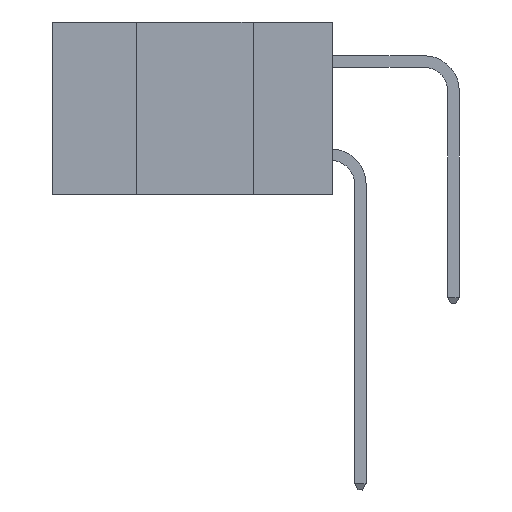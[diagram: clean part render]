
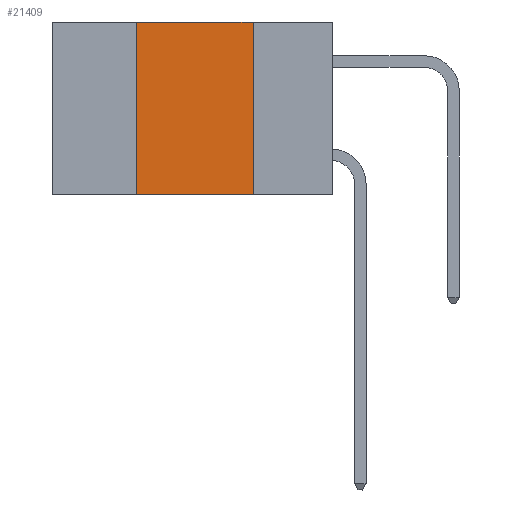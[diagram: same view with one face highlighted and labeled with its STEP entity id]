
A CAD part, left-side view. The second image highlights one B-rep face of the part: STEP entity #21409.
In plain terms, the highlighted planar face has unit normal (-1, 0, 0).
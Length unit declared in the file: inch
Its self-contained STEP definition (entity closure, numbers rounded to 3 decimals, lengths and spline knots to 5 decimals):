
#1539 = DIRECTION ( 'NONE',  ( 0., 0., -1. ) ) ;
#1586 = VERTEX_POINT ( 'NONE', #4110 ) ;
#3507 = ORIENTED_EDGE ( 'NONE', *, *, #20009, .F. ) ;
#4110 = CARTESIAN_POINT ( 'NONE',  ( 0., 0.42, -0.37 ) ) ;
#5303 = CARTESIAN_POINT ( 'NONE',  ( 0., 0.42, 0. ) ) ;
#6192 = ORIENTED_EDGE ( 'NONE', *, *, #22214, .F. ) ;
#6319 = VERTEX_POINT ( 'NONE', #9510 ) ;
#7118 = VECTOR ( 'NONE', #18454, 39.37008 ) ;
#7575 = CARTESIAN_POINT ( 'NONE',  ( 0., 0.6, 0. ) ) ;
#8699 = DIRECTION ( 'NONE',  ( 0., 0., 1. ) ) ;
#8933 = LINE ( 'NONE', #19924, #21434 ) ;
#9510 = CARTESIAN_POINT ( 'NONE',  ( 0., 0.17, -0.37 ) ) ;
#11011 = VERTEX_POINT ( 'NONE', #16668 ) ;
#11103 = DIRECTION ( 'NONE',  ( 0., 0., -1. ) ) ;
#11945 = VECTOR ( 'NONE', #15463, 39.37008 ) ;
#13098 = DIRECTION ( 'NONE',  ( 1., 0., 0. ) ) ;
#13252 = LINE ( 'NONE', #7575, #7118 ) ;
#13442 = VERTEX_POINT ( 'NONE', #5303 ) ;
#14113 = AXIS2_PLACEMENT_3D ( 'NONE', #14909, #13098, #1539 ) ;
#14863 = ORIENTED_EDGE ( 'NONE', *, *, #20947, .F. ) ;
#14909 = CARTESIAN_POINT ( 'NONE',  ( 0., 0.6, 0. ) ) ;
#15463 = DIRECTION ( 'NONE',  ( 0., -1., 0. ) ) ;
#15949 = EDGE_LOOP ( 'NONE', ( #14863, #3507, #6192, #23330 ) ) ;
#16400 = VECTOR ( 'NONE', #11103, 39.37008 ) ;
#16524 = EDGE_CURVE ( 'NONE', #1586, #6319, #16701, .T. ) ;
#16668 = CARTESIAN_POINT ( 'NONE',  ( 0., 0.17, 0. ) ) ;
#16670 = LINE ( 'NONE', #22083, #16400 ) ;
#16701 = LINE ( 'NONE', #17157, #11945 ) ;
#17157 = CARTESIAN_POINT ( 'NONE',  ( 0., 0.6, -0.37 ) ) ;
#18454 = DIRECTION ( 'NONE',  ( 0., -1., 0. ) ) ;
#18786 = FACE_OUTER_BOUND ( 'NONE', #15949, .T. ) ;
#19890 = PLANE ( 'NONE',  #14113 ) ;
#19924 = CARTESIAN_POINT ( 'NONE',  ( 0., 0.42, -0.37 ) ) ;
#20009 = EDGE_CURVE ( 'NONE', #13442, #11011, #13252, .T. ) ;
#20947 = EDGE_CURVE ( 'NONE', #11011, #6319, #16670, .T. ) ;
#21409 = ADVANCED_FACE ( 'NONE', ( #18786 ), #19890, .F. ) ;
#21434 = VECTOR ( 'NONE', #8699, 39.37008 ) ;
#22083 = CARTESIAN_POINT ( 'NONE',  ( 0., 0.17, -0.37 ) ) ;
#22214 = EDGE_CURVE ( 'NONE', #1586, #13442, #8933, .T. ) ;
#23330 = ORIENTED_EDGE ( 'NONE', *, *, #16524, .T. ) ;
